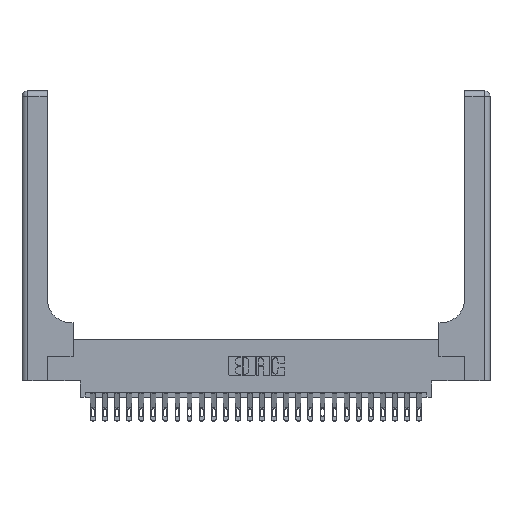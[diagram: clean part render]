
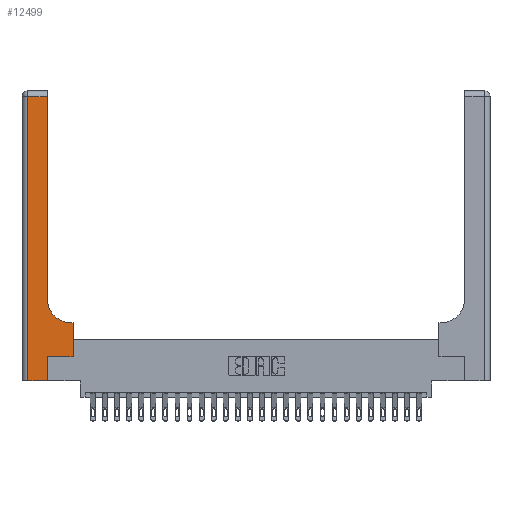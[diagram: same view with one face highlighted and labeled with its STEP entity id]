
A CAD part, top view. The second image highlights one B-rep face of the part: STEP entity #12499.
In plain terms, the highlighted planar face has unit normal (0, 0, 1).
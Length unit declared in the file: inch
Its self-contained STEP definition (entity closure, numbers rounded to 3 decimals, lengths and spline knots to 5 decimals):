
#166 = DIRECTION ( 'NONE',  ( 1., 0., 0. ) ) ;
#464 = ORIENTED_EDGE ( 'NONE', *, *, #7953, .T. ) ;
#856 = CARTESIAN_POINT ( 'NONE',  ( 0., 2.94, 0.37 ) ) ;
#1047 = CIRCLE ( 'NONE', #22265, 0.25 ) ;
#2324 = CARTESIAN_POINT ( 'NONE',  ( 0., 3., 0.37 ) ) ;
#2818 = LINE ( 'NONE', #12951, #12644 ) ;
#3122 = LINE ( 'NONE', #15130, #21813 ) ;
#3510 = ORIENTED_EDGE ( 'NONE', *, *, #24833, .T. ) ;
#4006 = LINE ( 'NONE', #24626, #26049 ) ;
#4015 = VECTOR ( 'NONE', #16617, 39.37008 ) ;
#4241 = CARTESIAN_POINT ( 'NONE',  ( 0., 0., 0.37 ) ) ;
#4469 = CARTESIAN_POINT ( 'NONE',  ( 0.265, 0.25, 0.37 ) ) ;
#4556 = VERTEX_POINT ( 'NONE', #19592 ) ;
#4983 = ORIENTED_EDGE ( 'NONE', *, *, #8557, .T. ) ;
#4985 = VECTOR ( 'NONE', #14793, 39.37008 ) ;
#5242 = CARTESIAN_POINT ( 'NONE',  ( 0.528, 0.6, 0.37 ) ) ;
#5580 = EDGE_CURVE ( 'NONE', #5865, #4556, #16493, .T. ) ;
#5865 = VERTEX_POINT ( 'NONE', #16072 ) ;
#6220 = LINE ( 'NONE', #14639, #6488 ) ;
#6260 = VECTOR ( 'NONE', #25195, 39.37008 ) ;
#6347 = DIRECTION ( 'NONE',  ( 0., 1., 0. ) ) ;
#6409 = ORIENTED_EDGE ( 'NONE', *, *, #22476, .T. ) ;
#6488 = VECTOR ( 'NONE', #6347, 39.37008 ) ;
#6516 = CARTESIAN_POINT ( 'NONE',  ( 0.528, 0.25, 0.37 ) ) ;
#6945 = LINE ( 'NONE', #856, #6260 ) ;
#6977 = CARTESIAN_POINT ( 'NONE',  ( 0.26, 0.85, 0.37 ) ) ;
#7058 = DIRECTION ( 'NONE',  ( 0., 1., 0. ) ) ;
#7156 = ORIENTED_EDGE ( 'NONE', *, *, #25499, .T. ) ;
#7953 = EDGE_CURVE ( 'NONE', #23015, #13513, #2818, .T. ) ;
#8557 = EDGE_CURVE ( 'NONE', #4556, #9146, #15188, .T. ) ;
#8630 = CARTESIAN_POINT ( 'NONE',  ( 0.265, 0., 0.37 ) ) ;
#9146 = VERTEX_POINT ( 'NONE', #4469 ) ;
#9795 = CARTESIAN_POINT ( 'NONE',  ( 0.51, 0.85, 0.37 ) ) ;
#10042 = DIRECTION ( 'NONE',  ( -1., 0., 0. ) ) ;
#10585 = PLANE ( 'NONE',  #22323 ) ;
#10886 = CARTESIAN_POINT ( 'NONE',  ( 0.51, 0.6, 0.37 ) ) ;
#11290 = DIRECTION ( 'NONE',  ( 1., 0., 0. ) ) ;
#11549 = DIRECTION ( 'NONE',  ( 0., 0., -1. ) ) ;
#12455 = FACE_OUTER_BOUND ( 'NONE', #16514, .T. ) ;
#12499 = ADVANCED_FACE ( 'NONE', ( #12455 ), #10585, .F. ) ;
#12644 = VECTOR ( 'NONE', #7058, 39.37008 ) ;
#12922 = EDGE_CURVE ( 'NONE', #13361, #19101, #24561, .T. ) ;
#12951 = CARTESIAN_POINT ( 'NONE',  ( 0.26, 3., 0.37 ) ) ;
#13153 = ORIENTED_EDGE ( 'NONE', *, *, #5580, .T. ) ;
#13361 = VERTEX_POINT ( 'NONE', #5242 ) ;
#13513 = VERTEX_POINT ( 'NONE', #15771 ) ;
#13785 = EDGE_CURVE ( 'NONE', #13513, #25925, #6945, .T. ) ;
#14472 = CARTESIAN_POINT ( 'NONE',  ( 0.26, 0.6, 0.37 ) ) ;
#14639 = CARTESIAN_POINT ( 'NONE',  ( 0.528, 0.25, 0.37 ) ) ;
#14793 = DIRECTION ( 'NONE',  ( 0., 1., 0. ) ) ;
#15063 = VECTOR ( 'NONE', #24286, 39.37008 ) ;
#15130 = CARTESIAN_POINT ( 'NONE',  ( 0.06, 3., 0.37 ) ) ;
#15188 = LINE ( 'NONE', #8630, #4985 ) ;
#15512 = ORIENTED_EDGE ( 'NONE', *, *, #13785, .T. ) ;
#15771 = CARTESIAN_POINT ( 'NONE',  ( 0.26, 2.94, 0.37 ) ) ;
#16072 = CARTESIAN_POINT ( 'NONE',  ( 0.06, 0., 0.37 ) ) ;
#16493 = LINE ( 'NONE', #4241, #4015 ) ;
#16514 = EDGE_LOOP ( 'NONE', ( #464, #15512, #18287, #13153, #4983, #3510, #6409, #20303, #7156 ) ) ;
#16617 = DIRECTION ( 'NONE',  ( 1., 0., 0. ) ) ;
#18287 = ORIENTED_EDGE ( 'NONE', *, *, #22941, .T. ) ;
#19101 = VERTEX_POINT ( 'NONE', #10886 ) ;
#19592 = CARTESIAN_POINT ( 'NONE',  ( 0.265, 0., 0.37 ) ) ;
#20303 = ORIENTED_EDGE ( 'NONE', *, *, #12922, .T. ) ;
#20827 = DIRECTION ( 'NONE',  ( 0., 0., -1. ) ) ;
#21813 = VECTOR ( 'NONE', #23100, 39.37008 ) ;
#22265 = AXIS2_PLACEMENT_3D ( 'NONE', #9795, #11549, #11290 ) ;
#22323 = AXIS2_PLACEMENT_3D ( 'NONE', #2324, #20827, #10042 ) ;
#22476 = EDGE_CURVE ( 'NONE', #24945, #13361, #6220, .T. ) ;
#22941 = EDGE_CURVE ( 'NONE', #25925, #5865, #3122, .T. ) ;
#23015 = VERTEX_POINT ( 'NONE', #6977 ) ;
#23100 = DIRECTION ( 'NONE',  ( 0., -1., 0. ) ) ;
#23232 = CARTESIAN_POINT ( 'NONE',  ( 0.06, 2.94, 0.37 ) ) ;
#24286 = DIRECTION ( 'NONE',  ( -1., 0., 0. ) ) ;
#24561 = LINE ( 'NONE', #14472, #15063 ) ;
#24626 = CARTESIAN_POINT ( 'NONE',  ( 0.265, 0.25, 0.37 ) ) ;
#24833 = EDGE_CURVE ( 'NONE', #9146, #24945, #4006, .T. ) ;
#24945 = VERTEX_POINT ( 'NONE', #6516 ) ;
#25195 = DIRECTION ( 'NONE',  ( -1., 0., 0. ) ) ;
#25499 = EDGE_CURVE ( 'NONE', #19101, #23015, #1047, .T. ) ;
#25925 = VERTEX_POINT ( 'NONE', #23232 ) ;
#26049 = VECTOR ( 'NONE', #166, 39.37008 ) ;
